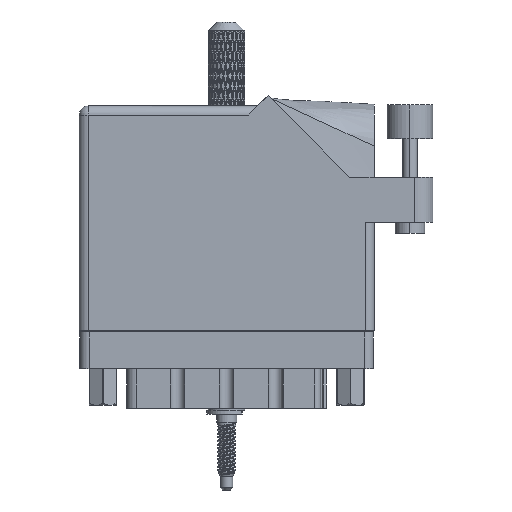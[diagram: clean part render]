
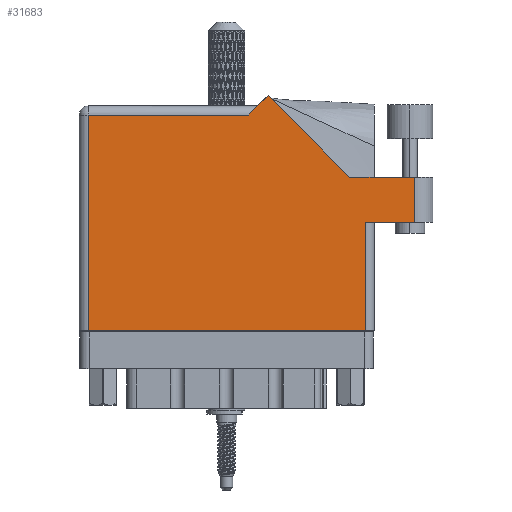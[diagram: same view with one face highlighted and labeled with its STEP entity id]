
A CAD part, front view. The second image highlights one B-rep face of the part: STEP entity #31683.
In plain terms, the highlighted face is planar.
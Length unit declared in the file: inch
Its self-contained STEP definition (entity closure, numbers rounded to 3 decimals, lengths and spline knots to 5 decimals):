
#1144 = CARTESIAN_POINT ( 'NONE',  ( 0., 1.468, 0. ) ) ;
#3030 = DIRECTION ( 'NONE',  ( -0.707, -0.707, 0. ) ) ;
#4196 = CARTESIAN_POINT ( 'NONE',  ( 1.217, 1.53, 0. ) ) ;
#5308 = DIRECTION ( 'NONE',  ( 0., 1., 0. ) ) ;
#6266 = AXIS2_PLACEMENT_3D ( 'NONE', #39952, #83805, #40356 ) ;
#6514 = VECTOR ( 'NONE', #49338, 39.37008 ) ;
#6611 = ORIENTED_EDGE ( 'NONE', *, *, #63662, .T. ) ;
#7610 = CARTESIAN_POINT ( 'NONE',  ( 0.062, 1.468, 0. ) ) ;
#8003 = ORIENTED_EDGE ( 'NONE', *, *, #17215, .T. ) ;
#8632 = LINE ( 'NONE', #104082, #11420 ) ;
#11420 = VECTOR ( 'NONE', #40760, 39.37008 ) ;
#12894 = DIRECTION ( 'NONE',  ( 1., 0., 0. ) ) ;
#12942 = CARTESIAN_POINT ( 'NONE',  ( 1.28771, 1.60071, 0. ) ) ;
#16226 = FACE_OUTER_BOUND ( 'NONE', #39453, .T. ) ;
#16322 = LINE ( 'NONE', #67018, #108519 ) ;
#17215 = EDGE_CURVE ( 'NONE', #29907, #53526, #60938, .T. ) ;
#18576 = LINE ( 'NONE', #48085, #26982 ) ;
#20492 = LINE ( 'NONE', #1144, #35808 ) ;
#21278 = PLANE ( 'NONE',  #6266 ) ;
#26428 = ORIENTED_EDGE ( 'NONE', *, *, #111500, .T. ) ;
#26982 = VECTOR ( 'NONE', #30509, 39.37008 ) ;
#28468 = CARTESIAN_POINT ( 'NONE',  ( 2.285, 0.737, 0. ) ) ;
#29907 = VERTEX_POINT ( 'NONE', #28468 ) ;
#30149 = CARTESIAN_POINT ( 'NONE',  ( 2.285, 1.044, 0. ) ) ;
#30509 = DIRECTION ( 'NONE',  ( 0., -1., 0. ) ) ;
#31348 = CARTESIAN_POINT ( 'NONE',  ( 2.41, 1.044, 0. ) ) ;
#31683 = ADVANCED_FACE ( 'NONE', ( #16226 ), #21278, .F. ) ;
#31866 = VECTOR ( 'NONE', #3030, 39.37008 ) ;
#35808 = VECTOR ( 'NONE', #62857, 39.37008 ) ;
#35989 = VERTEX_POINT ( 'NONE', #12942 ) ;
#37942 = VERTEX_POINT ( 'NONE', #71413 ) ;
#38250 = VERTEX_POINT ( 'NONE', #7610 ) ;
#38383 = VECTOR ( 'NONE', #92324, 39.37008 ) ;
#39138 = CARTESIAN_POINT ( 'NONE',  ( 2.01, 0.737, 0. ) ) ;
#39453 = EDGE_LOOP ( 'NONE', ( #92420, #8003, #57083, #75575, #110144, #69738, #54187, #6611, #26428 ) ) ;
#39820 = CARTESIAN_POINT ( 'NONE',  ( 1.155, 1.468, 0. ) ) ;
#39952 = CARTESIAN_POINT ( 'NONE',  ( 0., 1.53, 0. ) ) ;
#40356 = DIRECTION ( 'NONE',  ( -1., 0., 0. ) ) ;
#40760 = DIRECTION ( 'NONE',  ( -0.707, 0.707, 0. ) ) ;
#44424 = CARTESIAN_POINT ( 'NONE',  ( 2.285, 1.044, 0. ) ) ;
#46109 = CARTESIAN_POINT ( 'NONE',  ( 1.948, 0., 0. ) ) ;
#48085 = CARTESIAN_POINT ( 'NONE',  ( 0.062, 0., 0. ) ) ;
#49338 = DIRECTION ( 'NONE',  ( -1., 0., 0. ) ) ;
#49948 = CARTESIAN_POINT ( 'NONE',  ( 1.948, 0.737, 0. ) ) ;
#53526 = VERTEX_POINT ( 'NONE', #44424 ) ;
#54187 = ORIENTED_EDGE ( 'NONE', *, *, #73022, .T. ) ;
#56847 = VERTEX_POINT ( 'NONE', #39820 ) ;
#57083 = ORIENTED_EDGE ( 'NONE', *, *, #69789, .T. ) ;
#60938 = LINE ( 'NONE', #30149, #62366 ) ;
#61228 = EDGE_CURVE ( 'NONE', #35989, #56847, #79477, .T. ) ;
#62366 = VECTOR ( 'NONE', #101668, 39.37008 ) ;
#62857 = DIRECTION ( 'NONE',  ( -1., 0., 0. ) ) ;
#63662 = EDGE_CURVE ( 'NONE', #67171, #88039, #83272, .T. ) ;
#65564 = VERTEX_POINT ( 'NONE', #49948 ) ;
#67018 = CARTESIAN_POINT ( 'NONE',  ( 1.948, 0.737, 0. ) ) ;
#67171 = VERTEX_POINT ( 'NONE', #107690 ) ;
#69738 = ORIENTED_EDGE ( 'NONE', *, *, #102775, .T. ) ;
#69789 = EDGE_CURVE ( 'NONE', #53526, #37942, #83396, .T. ) ;
#71413 = CARTESIAN_POINT ( 'NONE',  ( 1.84442, 1.044, 0. ) ) ;
#73022 = EDGE_CURVE ( 'NONE', #38250, #67171, #18576, .T. ) ;
#75575 = ORIENTED_EDGE ( 'NONE', *, *, #95633, .T. ) ;
#79477 = LINE ( 'NONE', #4196, #31866 ) ;
#83272 = LINE ( 'NONE', #111992, #98593 ) ;
#83396 = LINE ( 'NONE', #31348, #6514 ) ;
#83805 = DIRECTION ( 'NONE',  ( 0., 0., -1. ) ) ;
#88039 = VERTEX_POINT ( 'NONE', #46109 ) ;
#92324 = DIRECTION ( 'NONE',  ( 1., 0., 0. ) ) ;
#92420 = ORIENTED_EDGE ( 'NONE', *, *, #104282, .T. ) ;
#92937 = LINE ( 'NONE', #39138, #38383 ) ;
#95633 = EDGE_CURVE ( 'NONE', #37942, #35989, #8632, .T. ) ;
#98593 = VECTOR ( 'NONE', #12894, 39.37008 ) ;
#101668 = DIRECTION ( 'NONE',  ( 0., 1., 0. ) ) ;
#102775 = EDGE_CURVE ( 'NONE', #56847, #38250, #20492, .T. ) ;
#104082 = CARTESIAN_POINT ( 'NONE',  ( 1.84442, 1.044, 0. ) ) ;
#104282 = EDGE_CURVE ( 'NONE', #65564, #29907, #92937, .T. ) ;
#107690 = CARTESIAN_POINT ( 'NONE',  ( 0.062, 0., 0. ) ) ;
#108519 = VECTOR ( 'NONE', #5308, 39.37008 ) ;
#110144 = ORIENTED_EDGE ( 'NONE', *, *, #61228, .T. ) ;
#111500 = EDGE_CURVE ( 'NONE', #88039, #65564, #16322, .T. ) ;
#111992 = CARTESIAN_POINT ( 'NONE',  ( 0., 0., 0. ) ) ;
